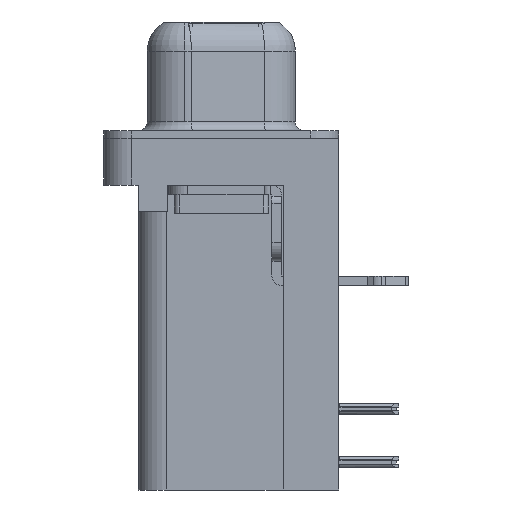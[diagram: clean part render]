
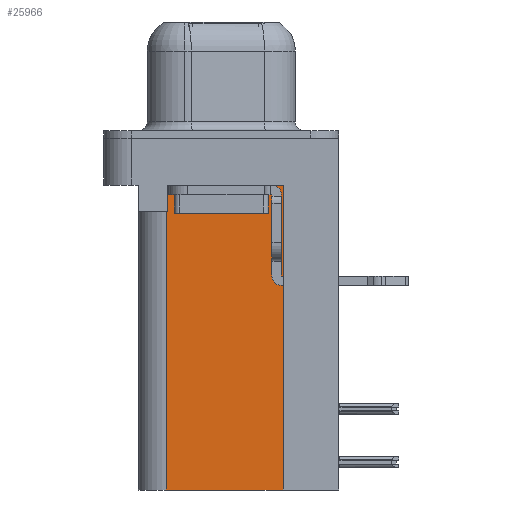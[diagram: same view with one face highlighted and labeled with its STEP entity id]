
A CAD part, left-side view. The second image highlights one B-rep face of the part: STEP entity #25966.
In plain terms, the highlighted planar face has unit normal (-1, 0, 0).
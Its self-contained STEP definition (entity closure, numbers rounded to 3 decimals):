
#123 = CARTESIAN_POINT ( 'NONE',  ( 3.79, -3.295, -2.5 ) ) ;
#317 = DIRECTION ( 'NONE',  ( 1., 0., 0. ) ) ;
#592 = AXIS2_PLACEMENT_3D ( 'NONE', #17298, #317, #20088 ) ;
#1188 = VERTEX_POINT ( 'NONE', #13745 ) ;
#1997 = EDGE_CURVE ( 'NONE', #27191, #1188, #20462, .T. ) ;
#2090 = VECTOR ( 'NONE', #31415, 1000. ) ;
#2163 = LINE ( 'NONE', #123, #2090 ) ;
#3190 = ORIENTED_EDGE ( 'NONE', *, *, #4594, .T. ) ;
#3440 = DIRECTION ( 'NONE',  ( 0., 0., -1. ) ) ;
#3880 = VECTOR ( 'NONE', #5823, 1000. ) ;
#3882 = CARTESIAN_POINT ( 'NONE',  ( 3.79, 0., -3.9 ) ) ;
#4173 = LINE ( 'NONE', #28497, #3880 ) ;
#4594 = EDGE_CURVE ( 'NONE', #29192, #27191, #2163, .T. ) ;
#5823 = DIRECTION ( 'NONE',  ( 0., 1., 0. ) ) ;
#6892 = ORIENTED_EDGE ( 'NONE', *, *, #1997, .T. ) ;
#7902 = EDGE_CURVE ( 'NONE', #24025, #12232, #21323, .T. ) ;
#8112 = ORIENTED_EDGE ( 'NONE', *, *, #16724, .F. ) ;
#10705 = VECTOR ( 'NONE', #20575, 1000. ) ;
#10746 = LINE ( 'NONE', #23211, #10705 ) ;
#11531 = PLANE ( 'NONE',  #592 ) ;
#12232 = VERTEX_POINT ( 'NONE', #22671 ) ;
#13745 = CARTESIAN_POINT ( 'NONE',  ( 3.79, 2.895, -3.9 ) ) ;
#15824 = ORIENTED_EDGE ( 'NONE', *, *, #24171, .T. ) ;
#16585 = ORIENTED_EDGE ( 'NONE', *, *, #26607, .T. ) ;
#16724 = EDGE_CURVE ( 'NONE', #31060, #24025, #4173, .T. ) ;
#17298 = CARTESIAN_POINT ( 'NONE',  ( 3.79, -3.295, -18.76 ) ) ;
#17557 = CARTESIAN_POINT ( 'NONE',  ( 3.79, -3.295, -18.76 ) ) ;
#18396 = VECTOR ( 'NONE', #23524, 1000. ) ;
#18465 = LINE ( 'NONE', #3882, #18396 ) ;
#20088 = DIRECTION ( 'NONE',  ( 0., 1., 0. ) ) ;
#20388 = VECTOR ( 'NONE', #3440, 1000. ) ;
#20462 = LINE ( 'NONE', #28748, #20388 ) ;
#20575 = DIRECTION ( 'NONE',  ( 0., 0., 1. ) ) ;
#20607 = EDGE_LOOP ( 'NONE', ( #3190, #6892, #16585, #26200, #8112, #15824 ) ) ;
#21323 = LINE ( 'NONE', #24666, #21419 ) ;
#21419 = VECTOR ( 'NONE', #27677, 1000. ) ;
#22671 = CARTESIAN_POINT ( 'NONE',  ( 3.79, 2.925, -3.9 ) ) ;
#23211 = CARTESIAN_POINT ( 'NONE',  ( 3.79, -3.295, -18.76 ) ) ;
#23524 = DIRECTION ( 'NONE',  ( 0., 1., 0. ) ) ;
#24025 = VERTEX_POINT ( 'NONE', #25575 ) ;
#24171 = EDGE_CURVE ( 'NONE', #31060, #29192, #10746, .T. ) ;
#24666 = CARTESIAN_POINT ( 'NONE',  ( 3.79, 2.925, -18.76 ) ) ;
#25575 = CARTESIAN_POINT ( 'NONE',  ( 3.79, 2.925, -18.76 ) ) ;
#25587 = CARTESIAN_POINT ( 'NONE',  ( 3.79, -3.295, -2.5 ) ) ;
#25883 = FACE_OUTER_BOUND ( 'NONE', #20607, .T. ) ;
#25966 = ADVANCED_FACE ( 'NONE', ( #25883 ), #11531, .F. ) ;
#26200 = ORIENTED_EDGE ( 'NONE', *, *, #7902, .F. ) ;
#26607 = EDGE_CURVE ( 'NONE', #1188, #12232, #18465, .T. ) ;
#27191 = VERTEX_POINT ( 'NONE', #29612 ) ;
#27677 = DIRECTION ( 'NONE',  ( 0., 0., 1. ) ) ;
#28497 = CARTESIAN_POINT ( 'NONE',  ( 3.79, -3.295, -18.76 ) ) ;
#28748 = CARTESIAN_POINT ( 'NONE',  ( 3.79, 2.895, -3.9 ) ) ;
#29192 = VERTEX_POINT ( 'NONE', #25587 ) ;
#29612 = CARTESIAN_POINT ( 'NONE',  ( 3.79, 2.895, -2.5 ) ) ;
#31060 = VERTEX_POINT ( 'NONE', #17557 ) ;
#31415 = DIRECTION ( 'NONE',  ( 0., 1., 0. ) ) ;
